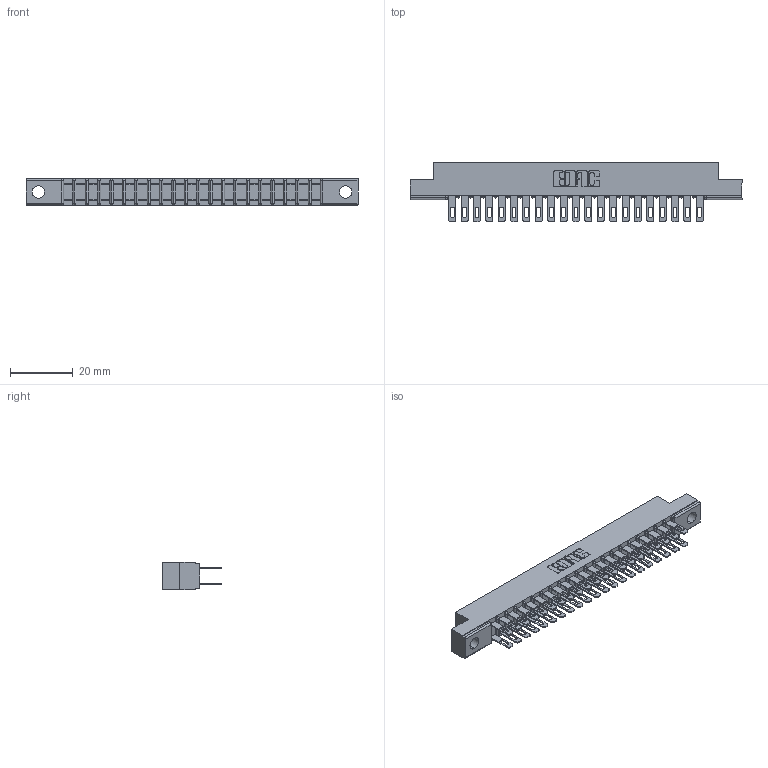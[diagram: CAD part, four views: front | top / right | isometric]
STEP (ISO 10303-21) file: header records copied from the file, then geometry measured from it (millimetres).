
FILE_DESCRIPTION (( 'STEP AP203' ), '1' );
FILE_NAME ('357-042-500-204.STEP', '2019-09-18T05:58:49', ( '' ), ( '' ), 'SwSTEP 2.0', 'SolidWorks 2016', '' );
FILE_SCHEMA (( 'CONFIG_CONTROL_DESIGN' ));
Length unit declared in the file: inch
Products named in the file (3): 307 Part_.156 Dia Mounting Holes; 307-290-001_500; 357-042-500-204
Assembly tree (43 placements, depth 2):
  357-042-500-204
    307 Part_.156 Dia Mounting Holes
    307-290-001_500  x42
Bounding box: 106.22 x 19.18 x 8.71 mm (x, y, z)
Volume: 6962.6 mm3; surface area: 12801.6 mm2
Topology: 43 solids, 43 shells, 2086 faces, 5819 edges, 3762 vertices
Faces by surface type: plane 1344, cylinder 698, sphere 44
Entity records: 21656 total; most frequent: CARTESIAN_POINT 3551, ORIENTED_EDGE 3514, DIRECTION 3481, EDGE_CURVE 1757, VECTOR 1345, LINE 1345, VERTEX_POINT 1138, AXIS2_PLACEMENT_3D 1068
